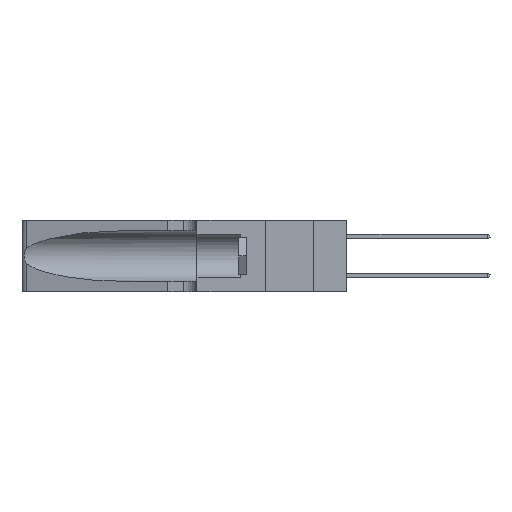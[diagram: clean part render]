
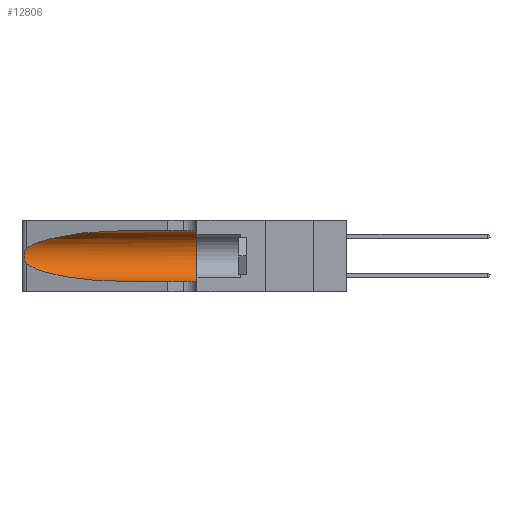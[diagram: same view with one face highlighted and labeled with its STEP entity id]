
A CAD part, left-side view. The second image highlights one B-rep face of the part: STEP entity #12806.
In plain terms, the highlighted cylindrical face has radius 3.308 mm (diameter 6.617 mm), a partial arc.
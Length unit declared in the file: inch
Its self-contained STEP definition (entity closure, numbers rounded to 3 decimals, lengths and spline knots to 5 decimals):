
#1752 = CARTESIAN_POINT ( 'NONE',  ( 0.25856, 1.23593, 0.16098 ) ) ;
#2211 =( BOUNDED_CURVE ( )  B_SPLINE_CURVE ( 3, ( #7467, #29812, #33523, #11259 ),
 .UNSPECIFIED., .F., .F. ) 
 B_SPLINE_CURVE_WITH_KNOTS ( ( 4, 4 ),
 ( 3.44316, 4.71239 ),
 .UNSPECIFIED. ) 
 CURVE ( )  GEOMETRIC_REPRESENTATION_ITEM ( )  RATIONAL_B_SPLINE_CURVE ( ( 1., 0.87, 0.87, 1. ) ) 
 REPRESENTATION_ITEM ( '' )  );
#4375 = CARTESIAN_POINT ( 'NONE',  ( 0.1305, 0.72297, 0.05475 ) ) ;
#5335 = CARTESIAN_POINT ( 'NONE',  ( 0.25487, 1.22718, 0.22369 ) ) ;
#5505 = CARTESIAN_POINT ( 'NONE',  ( 0.25639, 1.23186, 0.15144 ) ) ;
#5820 = EDGE_CURVE ( 'NONE', #21707, #15724, #17616, .T. ) ;
#6354 = EDGE_LOOP ( 'NONE', ( #20846, #18689, #19917, #46695, #28426, #36260 ) ) ;
#7467 = CARTESIAN_POINT ( 'NONE',  ( 0.25487, 1.22718, 0.14631 ) ) ;
#7569 = VERTEX_POINT ( 'NONE', #46819 ) ;
#7845 = CIRCLE ( 'NONE', #20864, 0.13025 ) ;
#8826 = VECTOR ( 'NONE', #43755, 39.37008 ) ;
#9272 = CARTESIAN_POINT ( 'NONE',  ( 0.25487, 1.22718, 0.14631 ) ) ;
#10786 = CARTESIAN_POINT ( 'NONE',  ( 0.1305, 0.72297, 0.31525 ) ) ;
#11259 = CARTESIAN_POINT ( 'NONE',  ( 0.1305, 0.72297, 0.05475 ) ) ;
#11705 = LINE ( 'NONE', #37692, #30339 ) ;
#12806 = ADVANCED_FACE ( 'NONE', ( #43747 ), #24058, .F. ) ;
#12858 = CARTESIAN_POINT ( 'NONE',  ( 0.25639, 1.23184, 0.21858 ) ) ;
#13394 = CARTESIAN_POINT ( 'NONE',  ( 0.1305, 1.61858, 0.185 ) ) ;
#14355 = CARTESIAN_POINT ( 'NONE',  ( 0.18966, 0.96281, 0.31525 ) ) ;
#14559 = AXIS2_PLACEMENT_3D ( 'NONE', #13394, #46435, #35626 ) ;
#15724 = VERTEX_POINT ( 'NONE', #31766 ) ;
#15904 = EDGE_CURVE ( 'NONE', #34226, #27546, #2211, .T. ) ;
#16205 = EDGE_CURVE ( 'NONE', #7569, #34226, #41855, .T. ) ;
#16626 = CARTESIAN_POINT ( 'NONE',  ( 0.25854, 1.2359, 0.20912 ) ) ;
#17616 = LINE ( 'NONE', #17867, #8826 ) ;
#17867 = CARTESIAN_POINT ( 'NONE',  ( 0.1305, 1.61858, 0.31525 ) ) ;
#18295 = CARTESIAN_POINT ( 'NONE',  ( 0.2373, 1.15595, 0.28018 ) ) ;
#18689 = ORIENTED_EDGE ( 'NONE', *, *, #16205, .T. ) ;
#19917 = ORIENTED_EDGE ( 'NONE', *, *, #15904, .T. ) ;
#20378 = CARTESIAN_POINT ( 'NONE',  ( 0.26075, 1.23896, 0.19203 ) ) ;
#20846 = ORIENTED_EDGE ( 'NONE', *, *, #44593, .T. ) ;
#20864 = AXIS2_PLACEMENT_3D ( 'NONE', #21970, #47828, #25688 ) ;
#21087 =( BOUNDED_CURVE ( )  B_SPLINE_CURVE ( 3, ( #10786, #14355, #18295, #44180 ),
 .UNSPECIFIED., .F., .F. ) 
 B_SPLINE_CURVE_WITH_KNOTS ( ( 4, 4 ),
 ( 1.5708, 2.84003 ),
 .UNSPECIFIED. ) 
 CURVE ( )  GEOMETRIC_REPRESENTATION_ITEM ( )  RATIONAL_B_SPLINE_CURVE ( ( 1., 0.87, 0.87, 1. ) ) 
 REPRESENTATION_ITEM ( '' )  );
#21707 = VERTEX_POINT ( 'NONE', #35311 ) ;
#21970 = CARTESIAN_POINT ( 'NONE',  ( 0.1305, 0.35, 0.185 ) ) ;
#24058 = CYLINDRICAL_SURFACE ( 'NONE', #14559, 0.13025 ) ;
#24082 = CARTESIAN_POINT ( 'NONE',  ( 0.26017, 1.23833, 0.17102 ) ) ;
#24304 = VERTEX_POINT ( 'NONE', #46904 ) ;
#25688 = DIRECTION ( 'NONE',  ( 0., 0., 1. ) ) ;
#27546 = VERTEX_POINT ( 'NONE', #4375 ) ;
#27690 = CARTESIAN_POINT ( 'NONE',  ( 0.25555, 1.22994, 0.2215 ) ) ;
#27861 = CARTESIAN_POINT ( 'NONE',  ( 0.25789, 1.23486, 0.15765 ) ) ;
#28426 = ORIENTED_EDGE ( 'NONE', *, *, #36910, .F. ) ;
#29812 = CARTESIAN_POINT ( 'NONE',  ( 0.2373, 1.15595, 0.08982 ) ) ;
#30339 = VECTOR ( 'NONE', #41399, 39.37008 ) ;
#30997 = EDGE_CURVE ( 'NONE', #27546, #24304, #11705, .T. ) ;
#31565 = CARTESIAN_POINT ( 'NONE',  ( 0.25555, 1.22993, 0.14849 ) ) ;
#31766 = CARTESIAN_POINT ( 'NONE',  ( 0.1305, 0.35, 0.31525 ) ) ;
#33523 = CARTESIAN_POINT ( 'NONE',  ( 0.18966, 0.96281, 0.05475 ) ) ;
#34226 = VERTEX_POINT ( 'NONE', #36953 ) ;
#35311 = CARTESIAN_POINT ( 'NONE',  ( 0.1305, 0.72297, 0.31525 ) ) ;
#35626 = DIRECTION ( 'NONE',  ( 0., 0., -1. ) ) ;
#36260 = ORIENTED_EDGE ( 'NONE', *, *, #5820, .F. ) ;
#36910 = EDGE_CURVE ( 'NONE', #15724, #24304, #7845, .T. ) ;
#36953 = CARTESIAN_POINT ( 'NONE',  ( 0.25487, 1.22718, 0.14631 ) ) ;
#37692 = CARTESIAN_POINT ( 'NONE',  ( 0.1305, 1.61858, 0.05475 ) ) ;
#38886 = CARTESIAN_POINT ( 'NONE',  ( 0.25787, 1.23484, 0.2124 ) ) ;
#41399 = DIRECTION ( 'NONE',  ( 0., -1., 0. ) ) ;
#41855 = B_SPLINE_CURVE_WITH_KNOTS ( 'NONE', 3,
 ( #5335, #27690, #12858, #38886, #16626, #42543, #20378, #46247, #24082, #1752, #27861, #5505, #31565, #9272 ),
 .UNSPECIFIED., .F., .F.,
 ( 4, 2, 2, 2, 2, 2, 4 ),
 ( 0., 0.00027, 0.00053, 0.00107, 0.0016, 0.00187, 0.00214 ),
 .UNSPECIFIED. ) ;
#42543 = CARTESIAN_POINT ( 'NONE',  ( 0.26018, 1.23835, 0.19895 ) ) ;
#43747 = FACE_OUTER_BOUND ( 'NONE', #6354, .T. ) ;
#43755 = DIRECTION ( 'NONE',  ( 0., -1., 0. ) ) ;
#44180 = CARTESIAN_POINT ( 'NONE',  ( 0.25487, 1.22718, 0.22369 ) ) ;
#44593 = EDGE_CURVE ( 'NONE', #21707, #7569, #21087, .T. ) ;
#46247 = CARTESIAN_POINT ( 'NONE',  ( 0.26075, 1.23896, 0.178 ) ) ;
#46435 = DIRECTION ( 'NONE',  ( 0., -1., 0. ) ) ;
#46695 = ORIENTED_EDGE ( 'NONE', *, *, #30997, .T. ) ;
#46819 = CARTESIAN_POINT ( 'NONE',  ( 0.25487, 1.22718, 0.22369 ) ) ;
#46904 = CARTESIAN_POINT ( 'NONE',  ( 0.1305, 0.35, 0.05475 ) ) ;
#47828 = DIRECTION ( 'NONE',  ( 0., 1., 0. ) ) ;
